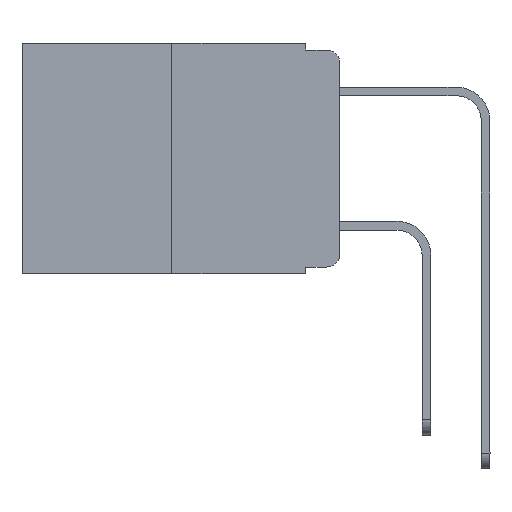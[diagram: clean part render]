
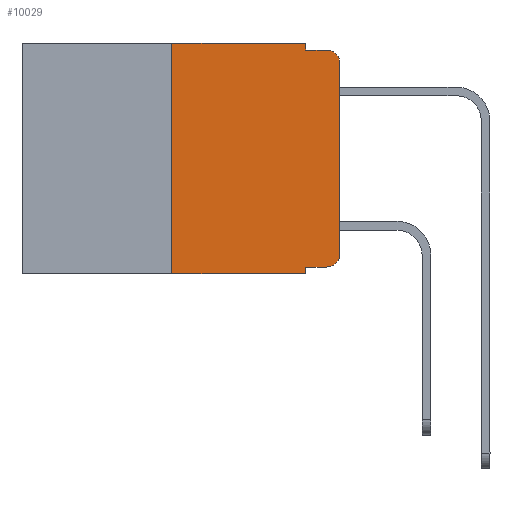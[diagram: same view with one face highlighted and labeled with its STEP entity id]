
A CAD part, left-side view. The second image highlights one B-rep face of the part: STEP entity #10029.
In plain terms, the highlighted planar face has unit normal (-1, 0, 0).
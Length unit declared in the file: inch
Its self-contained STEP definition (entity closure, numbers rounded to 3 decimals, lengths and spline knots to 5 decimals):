
#89 = DIRECTION ( 'NONE',  ( 0., -1., 0. ) ) ;
#134 = DIRECTION ( 'NONE',  ( -1., 0., 0. ) ) ;
#240 = ORIENTED_EDGE ( 'NONE', *, *, #9362, .T. ) ;
#585 = ORIENTED_EDGE ( 'NONE', *, *, #12322, .T. ) ;
#603 = CARTESIAN_POINT ( 'NONE',  ( 0., 0.051, 0. ) ) ;
#615 = VECTOR ( 'NONE', #13385, 39.37008 ) ;
#650 = CARTESIAN_POINT ( 'NONE',  ( 0., 0.051, 0. ) ) ;
#918 = VECTOR ( 'NONE', #7831, 39.37008 ) ;
#1083 = CARTESIAN_POINT ( 'NONE',  ( 0., 0.25, 0. ) ) ;
#1654 = ORIENTED_EDGE ( 'NONE', *, *, #12464, .F. ) ;
#2133 = CIRCLE ( 'NONE', #14636, 0.02 ) ;
#2302 = CARTESIAN_POINT ( 'NONE',  ( 0., 0.051, -0.01 ) ) ;
#2417 = DIRECTION ( 'NONE',  ( 0., 0., -1. ) ) ;
#2571 = EDGE_CURVE ( 'NONE', #9097, #10349, #3676, .T. ) ;
#2783 = CARTESIAN_POINT ( 'NONE',  ( 0., 0.02, -0.333 ) ) ;
#2903 = ORIENTED_EDGE ( 'NONE', *, *, #10984, .T. ) ;
#3664 = VECTOR ( 'NONE', #15180, 39.37008 ) ;
#3676 = LINE ( 'NONE', #4929, #13950 ) ;
#3831 = CARTESIAN_POINT ( 'NONE',  ( 0., 0.02, -0.313 ) ) ;
#4049 = VERTEX_POINT ( 'NONE', #8847 ) ;
#4067 = CARTESIAN_POINT ( 'NONE',  ( 0., 0., -0.313 ) ) ;
#4097 = LINE ( 'NONE', #8807, #6963 ) ;
#4597 = CARTESIAN_POINT ( 'NONE',  ( 0., 0.25, 0. ) ) ;
#4929 = CARTESIAN_POINT ( 'NONE',  ( 0., 0., 0. ) ) ;
#5063 = VERTEX_POINT ( 'NONE', #5116 ) ;
#5116 = CARTESIAN_POINT ( 'NONE',  ( 0., 0.051, -0.01 ) ) ;
#5122 = EDGE_CURVE ( 'NONE', #14614, #5063, #11651, .T. ) ;
#5305 = CARTESIAN_POINT ( 'NONE',  ( 0., 0., -0.03 ) ) ;
#5444 = LINE ( 'NONE', #13853, #3664 ) ;
#5574 = CARTESIAN_POINT ( 'NONE',  ( 0., 0.051, 0. ) ) ;
#5798 = EDGE_LOOP ( 'NONE', ( #7572, #240, #6753, #11264, #15169, #10543, #2903, #1654, #6975, #585 ) ) ;
#6381 = VERTEX_POINT ( 'NONE', #2783 ) ;
#6456 = CARTESIAN_POINT ( 'NONE',  ( 0., 0.25, -0.343 ) ) ;
#6753 = ORIENTED_EDGE ( 'NONE', *, *, #7152, .F. ) ;
#6773 = DIRECTION ( 'NONE',  ( 0., 0., 1. ) ) ;
#6963 = VECTOR ( 'NONE', #8881, 39.37008 ) ;
#6975 = ORIENTED_EDGE ( 'NONE', *, *, #14603, .T. ) ;
#7019 = VECTOR ( 'NONE', #7876, 39.37008 ) ;
#7109 = DIRECTION ( 'NONE',  ( -1., 0., 0. ) ) ;
#7152 = EDGE_CURVE ( 'NONE', #5063, #4049, #10938, .T. ) ;
#7504 = CARTESIAN_POINT ( 'NONE',  ( 0., 0.473, 0. ) ) ;
#7572 = ORIENTED_EDGE ( 'NONE', *, *, #2571, .T. ) ;
#7588 = CARTESIAN_POINT ( 'NONE',  ( 0., 0.051, -0.343 ) ) ;
#7831 = DIRECTION ( 'NONE',  ( 0., 0., -1. ) ) ;
#7876 = DIRECTION ( 'NONE',  ( 0., 0., -1. ) ) ;
#8178 = AXIS2_PLACEMENT_3D ( 'NONE', #3831, #134, #8610 ) ;
#8517 = CARTESIAN_POINT ( 'NONE',  ( 0., 0.473, 0. ) ) ;
#8610 = DIRECTION ( 'NONE',  ( 0., 0., -1. ) ) ;
#8794 = VERTEX_POINT ( 'NONE', #9273 ) ;
#8807 = CARTESIAN_POINT ( 'NONE',  ( 0., 0.051, -0.333 ) ) ;
#8847 = CARTESIAN_POINT ( 'NONE',  ( 0., 0.02, -0.01 ) ) ;
#8881 = DIRECTION ( 'NONE',  ( 0., -1., 0. ) ) ;
#9076 = LINE ( 'NONE', #603, #918 ) ;
#9097 = VERTEX_POINT ( 'NONE', #4067 ) ;
#9273 = CARTESIAN_POINT ( 'NONE',  ( 0., 0.051, -0.333 ) ) ;
#9316 = LINE ( 'NONE', #4597, #13399 ) ;
#9362 = EDGE_CURVE ( 'NONE', #10349, #4049, #2133, .T. ) ;
#9447 = VERTEX_POINT ( 'NONE', #1083 ) ;
#9493 = EDGE_CURVE ( 'NONE', #9447, #14614, #14564, .T. ) ;
#9695 = FACE_OUTER_BOUND ( 'NONE', #5798, .T. ) ;
#10029 = ADVANCED_FACE ( 'NONE', ( #9695 ), #14470, .F. ) ;
#10349 = VERTEX_POINT ( 'NONE', #5305 ) ;
#10543 = ORIENTED_EDGE ( 'NONE', *, *, #11143, .F. ) ;
#10676 = DIRECTION ( 'NONE',  ( 0., 0., 1. ) ) ;
#10746 = CARTESIAN_POINT ( 'NONE',  ( 0., 0.02, -0.03 ) ) ;
#10938 = LINE ( 'NONE', #2302, #14826 ) ;
#10984 = EDGE_CURVE ( 'NONE', #11091, #12420, #5444, .T. ) ;
#11091 = VERTEX_POINT ( 'NONE', #6456 ) ;
#11143 = EDGE_CURVE ( 'NONE', #11091, #9447, #9316, .T. ) ;
#11161 = AXIS2_PLACEMENT_3D ( 'NONE', #8517, #13365, #13300 ) ;
#11264 = ORIENTED_EDGE ( 'NONE', *, *, #5122, .F. ) ;
#11651 = LINE ( 'NONE', #5574, #7019 ) ;
#12322 = EDGE_CURVE ( 'NONE', #6381, #9097, #14669, .T. ) ;
#12420 = VERTEX_POINT ( 'NONE', #7588 ) ;
#12464 = EDGE_CURVE ( 'NONE', #8794, #12420, #9076, .T. ) ;
#13300 = DIRECTION ( 'NONE',  ( 0., 0., -1. ) ) ;
#13365 = DIRECTION ( 'NONE',  ( 1., 0., 0. ) ) ;
#13385 = DIRECTION ( 'NONE',  ( 0., -1., 0. ) ) ;
#13399 = VECTOR ( 'NONE', #6773, 39.37008 ) ;
#13853 = CARTESIAN_POINT ( 'NONE',  ( 0., 0.473, -0.343 ) ) ;
#13950 = VECTOR ( 'NONE', #10676, 39.37008 ) ;
#14470 = PLANE ( 'NONE',  #11161 ) ;
#14564 = LINE ( 'NONE', #7504, #615 ) ;
#14603 = EDGE_CURVE ( 'NONE', #8794, #6381, #4097, .T. ) ;
#14614 = VERTEX_POINT ( 'NONE', #650 ) ;
#14636 = AXIS2_PLACEMENT_3D ( 'NONE', #10746, #7109, #2417 ) ;
#14669 = CIRCLE ( 'NONE', #8178, 0.02 ) ;
#14826 = VECTOR ( 'NONE', #89, 39.37008 ) ;
#15169 = ORIENTED_EDGE ( 'NONE', *, *, #9493, .F. ) ;
#15180 = DIRECTION ( 'NONE',  ( 0., -1., 0. ) ) ;
